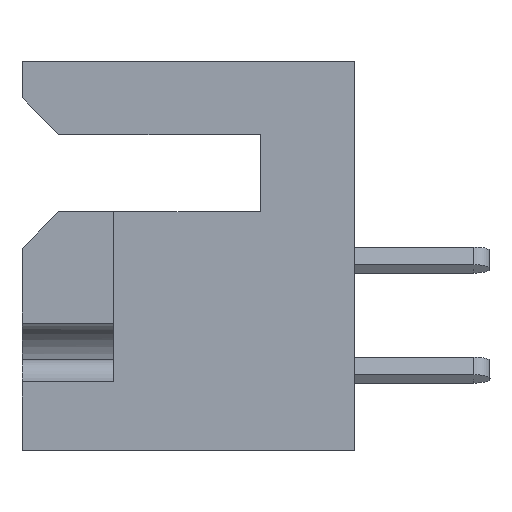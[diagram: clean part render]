
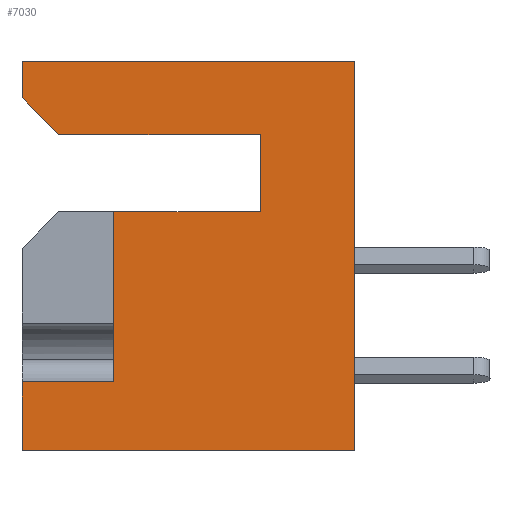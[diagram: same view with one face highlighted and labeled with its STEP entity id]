
A CAD part, left-side view. The second image highlights one B-rep face of the part: STEP entity #7030.
In plain terms, the highlighted planar face has unit normal (-1, 0, 0).
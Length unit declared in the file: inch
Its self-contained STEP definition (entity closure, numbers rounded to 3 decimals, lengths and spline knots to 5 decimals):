
#241 = DIRECTION ( 'NONE',  ( 0., 1., 0. ) ) ;
#522 = VERTEX_POINT ( 'NONE', #12105 ) ;
#539 = EDGE_CURVE ( 'NONE', #6186, #7858, #31993, .T. ) ;
#1558 = CARTESIAN_POINT ( 'NONE',  ( 0., 0.328, -0.205 ) ) ;
#1876 = VECTOR ( 'NONE', #24784, 39.37008 ) ;
#2334 = CARTESIAN_POINT ( 'NONE',  ( 0., 0.403, -0.1 ) ) ;
#2954 = CARTESIAN_POINT ( 'NONE',  ( 0., 0.128, -0.1 ) ) ;
#3238 = LINE ( 'NONE', #21069, #14142 ) ;
#3716 = CARTESIAN_POINT ( 'NONE',  ( 0., 0.453, -0.531 ) ) ;
#4048 = VERTEX_POINT ( 'NONE', #26419 ) ;
#4765 = ORIENTED_EDGE ( 'NONE', *, *, #19042, .T. ) ;
#4872 = ORIENTED_EDGE ( 'NONE', *, *, #22836, .T. ) ;
#5461 = PLANE ( 'NONE',  #26736 ) ;
#5532 = CARTESIAN_POINT ( 'NONE',  ( 0., 0.453, 0. ) ) ;
#5807 = VECTOR ( 'NONE', #15362, 39.37008 ) ;
#5962 = EDGE_CURVE ( 'NONE', #21475, #4048, #21266, .T. ) ;
#6186 = VERTEX_POINT ( 'NONE', #3716 ) ;
#6329 = VECTOR ( 'NONE', #10485, 39.37008 ) ;
#7030 = ADVANCED_FACE ( 'NONE', ( #32027 ), #5461, .F. ) ;
#7174 = DIRECTION ( 'NONE',  ( 0., 0., 1. ) ) ;
#7455 = ORIENTED_EDGE ( 'NONE', *, *, #5962, .T. ) ;
#7858 = VERTEX_POINT ( 'NONE', #11029 ) ;
#8165 = DIRECTION ( 'NONE',  ( 1., 0., 0. ) ) ;
#8877 = LINE ( 'NONE', #24703, #20169 ) ;
#8936 = LINE ( 'NONE', #10512, #5807 ) ;
#9970 = EDGE_CURVE ( 'NONE', #28679, #25621, #19593, .T. ) ;
#9995 = VECTOR ( 'NONE', #20367, 39.37008 ) ;
#10435 = VECTOR ( 'NONE', #241, 39.37008 ) ;
#10485 = DIRECTION ( 'NONE',  ( 0., 0., 1. ) ) ;
#10512 = CARTESIAN_POINT ( 'NONE',  ( 0., 0.453, 0. ) ) ;
#10708 = CARTESIAN_POINT ( 'NONE',  ( 0., 0., -0.531 ) ) ;
#11029 = CARTESIAN_POINT ( 'NONE',  ( 0., 0.453, -0.437 ) ) ;
#12105 = CARTESIAN_POINT ( 'NONE',  ( 0., 0.328, -0.437 ) ) ;
#12373 = ORIENTED_EDGE ( 'NONE', *, *, #22574, .F. ) ;
#13078 = ORIENTED_EDGE ( 'NONE', *, *, #19342, .F. ) ;
#13440 = VECTOR ( 'NONE', #17162, 39.37008 ) ;
#13762 = VECTOR ( 'NONE', #14333, 39.37008 ) ;
#14142 = VECTOR ( 'NONE', #30877, 39.37008 ) ;
#14333 = DIRECTION ( 'NONE',  ( 0., 0., 1. ) ) ;
#14473 = CARTESIAN_POINT ( 'NONE',  ( 0., 0.453, -0.05 ) ) ;
#14822 = VERTEX_POINT ( 'NONE', #15369 ) ;
#15362 = DIRECTION ( 'NONE',  ( 0., -1., 0. ) ) ;
#15369 = CARTESIAN_POINT ( 'NONE',  ( 0., 0.128, -0.1 ) ) ;
#15506 = CARTESIAN_POINT ( 'NONE',  ( 0., 0.453, 0. ) ) ;
#16305 = LINE ( 'NONE', #25001, #1876 ) ;
#16843 = CARTESIAN_POINT ( 'NONE',  ( 0., 0.128, -0.205 ) ) ;
#16890 = LINE ( 'NONE', #16843, #25385 ) ;
#17142 = EDGE_CURVE ( 'NONE', #21475, #21999, #22572, .T. ) ;
#17162 = DIRECTION ( 'NONE',  ( 0., -0.707, -0.707 ) ) ;
#17165 = CARTESIAN_POINT ( 'NONE',  ( 0., 0.453, 0. ) ) ;
#17395 = EDGE_CURVE ( 'NONE', #21999, #25621, #8936, .T. ) ;
#17498 = LINE ( 'NONE', #22744, #10435 ) ;
#18539 = ORIENTED_EDGE ( 'NONE', *, *, #18620, .T. ) ;
#18598 = CARTESIAN_POINT ( 'NONE',  ( 0., 0., 0. ) ) ;
#18620 = EDGE_CURVE ( 'NONE', #522, #7858, #17498, .T. ) ;
#19042 = EDGE_CURVE ( 'NONE', #6186, #28679, #8877, .T. ) ;
#19342 = EDGE_CURVE ( 'NONE', #14822, #4048, #24418, .T. ) ;
#19593 = LINE ( 'NONE', #27756, #6329 ) ;
#19598 = CARTESIAN_POINT ( 'NONE',  ( 0., 0.453, 0. ) ) ;
#20169 = VECTOR ( 'NONE', #21894, 39.37008 ) ;
#20367 = DIRECTION ( 'NONE',  ( 0., 1., 0. ) ) ;
#20569 = ORIENTED_EDGE ( 'NONE', *, *, #25342, .F. ) ;
#21069 = CARTESIAN_POINT ( 'NONE',  ( 0., 0.128, -0.1 ) ) ;
#21266 = LINE ( 'NONE', #2334, #13440 ) ;
#21475 = VERTEX_POINT ( 'NONE', #14473 ) ;
#21718 = ORIENTED_EDGE ( 'NONE', *, *, #17395, .F. ) ;
#21730 = ORIENTED_EDGE ( 'NONE', *, *, #539, .F. ) ;
#21825 = VERTEX_POINT ( 'NONE', #1558 ) ;
#21894 = DIRECTION ( 'NONE',  ( 0., -1., 0. ) ) ;
#21999 = VERTEX_POINT ( 'NONE', #5532 ) ;
#22572 = LINE ( 'NONE', #19598, #27985 ) ;
#22574 = EDGE_CURVE ( 'NONE', #28716, #14822, #3238, .T. ) ;
#22744 = CARTESIAN_POINT ( 'NONE',  ( 0., 0.328, -0.437 ) ) ;
#22836 = EDGE_CURVE ( 'NONE', #28716, #21825, #16890, .T. ) ;
#23010 = ORIENTED_EDGE ( 'NONE', *, *, #17142, .F. ) ;
#24418 = LINE ( 'NONE', #2954, #9995 ) ;
#24703 = CARTESIAN_POINT ( 'NONE',  ( 0., 0.453, -0.531 ) ) ;
#24784 = DIRECTION ( 'NONE',  ( 0., 0., 1. ) ) ;
#25001 = CARTESIAN_POINT ( 'NONE',  ( 0., 0.328, -0.205 ) ) ;
#25342 = EDGE_CURVE ( 'NONE', #522, #21825, #16305, .T. ) ;
#25385 = VECTOR ( 'NONE', #31413, 39.37008 ) ;
#25621 = VERTEX_POINT ( 'NONE', #18598 ) ;
#25663 = EDGE_LOOP ( 'NONE', ( #18539, #21730, #4765, #25990, #21718, #23010, #7455, #13078, #12373, #4872, #20569 ) ) ;
#25990 = ORIENTED_EDGE ( 'NONE', *, *, #9970, .T. ) ;
#26419 = CARTESIAN_POINT ( 'NONE',  ( 0., 0.403, -0.1 ) ) ;
#26736 = AXIS2_PLACEMENT_3D ( 'NONE', #15506, #8165, #28028 ) ;
#27756 = CARTESIAN_POINT ( 'NONE',  ( 0., 0., 0. ) ) ;
#27985 = VECTOR ( 'NONE', #7174, 39.37008 ) ;
#28028 = DIRECTION ( 'NONE',  ( 0., 0., -1. ) ) ;
#28679 = VERTEX_POINT ( 'NONE', #10708 ) ;
#28716 = VERTEX_POINT ( 'NONE', #29813 ) ;
#29813 = CARTESIAN_POINT ( 'NONE',  ( 0., 0.128, -0.205 ) ) ;
#30877 = DIRECTION ( 'NONE',  ( 0., 0., 1. ) ) ;
#31413 = DIRECTION ( 'NONE',  ( 0., 1., 0. ) ) ;
#31993 = LINE ( 'NONE', #17165, #13762 ) ;
#32027 = FACE_OUTER_BOUND ( 'NONE', #25663, .T. ) ;
